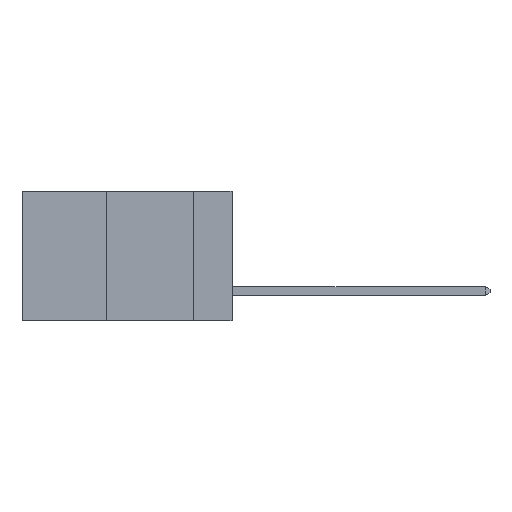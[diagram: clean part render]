
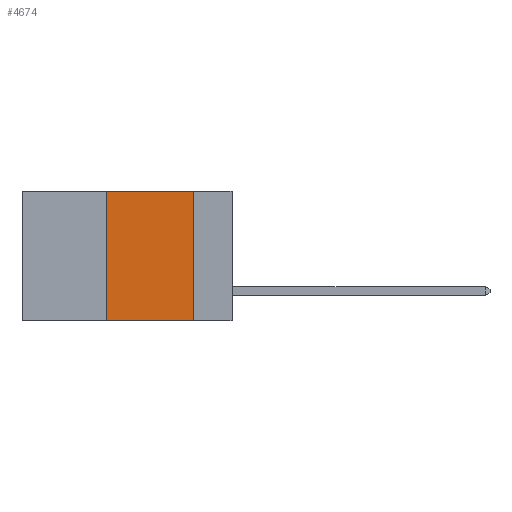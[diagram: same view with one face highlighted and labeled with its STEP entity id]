
A CAD part, left-side view. The second image highlights one B-rep face of the part: STEP entity #4674.
In plain terms, the highlighted planar face has unit normal (-1, 0, 0).
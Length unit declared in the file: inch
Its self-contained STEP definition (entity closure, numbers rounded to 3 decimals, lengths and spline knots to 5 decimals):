
#524 = VECTOR ( 'NONE', #16041, 39.37008 ) ;
#642 = EDGE_CURVE ( 'NONE', #1489, #13528, #15472, .T. ) ;
#1094 = EDGE_LOOP ( 'NONE', ( #17589, #17293, #4717, #20922 ) ) ;
#1489 = VERTEX_POINT ( 'NONE', #21468 ) ;
#2473 = AXIS2_PLACEMENT_3D ( 'NONE', #7374, #22878, #11309 ) ;
#3033 = CARTESIAN_POINT ( 'NONE',  ( 0., 0.36, 0. ) ) ;
#4674 = ADVANCED_FACE ( 'NONE', ( #10718 ), #20958, .F. ) ;
#4717 = ORIENTED_EDGE ( 'NONE', *, *, #10222, .F. ) ;
#4880 = CARTESIAN_POINT ( 'NONE',  ( 0., 0.36, 0. ) ) ;
#4892 = CARTESIAN_POINT ( 'NONE',  ( 0., 0.11, 0. ) ) ;
#5175 = VERTEX_POINT ( 'NONE', #4880 ) ;
#5497 = LINE ( 'NONE', #3033, #10768 ) ;
#5903 = LINE ( 'NONE', #14131, #524 ) ;
#7374 = CARTESIAN_POINT ( 'NONE',  ( 0., 0.6, 0. ) ) ;
#8728 = EDGE_CURVE ( 'NONE', #5175, #10208, #5903, .T. ) ;
#8800 = LINE ( 'NONE', #15427, #13407 ) ;
#9700 = VECTOR ( 'NONE', #23772, 39.37008 ) ;
#10208 = VERTEX_POINT ( 'NONE', #4892 ) ;
#10222 = EDGE_CURVE ( 'NONE', #1489, #5175, #5497, .T. ) ;
#10718 = FACE_OUTER_BOUND ( 'NONE', #1094, .T. ) ;
#10768 = VECTOR ( 'NONE', #14893, 39.37008 ) ;
#11309 = DIRECTION ( 'NONE',  ( 0., 0., -1. ) ) ;
#11674 = DIRECTION ( 'NONE',  ( 0., 0., -1. ) ) ;
#13407 = VECTOR ( 'NONE', #11674, 39.37008 ) ;
#13528 = VERTEX_POINT ( 'NONE', #15564 ) ;
#14131 = CARTESIAN_POINT ( 'NONE',  ( 0., 0.6, 0. ) ) ;
#14893 = DIRECTION ( 'NONE',  ( 0., 0., 1. ) ) ;
#15427 = CARTESIAN_POINT ( 'NONE',  ( 0., 0.11, 0. ) ) ;
#15445 = EDGE_CURVE ( 'NONE', #10208, #13528, #8800, .T. ) ;
#15472 = LINE ( 'NONE', #23644, #9700 ) ;
#15564 = CARTESIAN_POINT ( 'NONE',  ( 0., 0.11, -0.37 ) ) ;
#16041 = DIRECTION ( 'NONE',  ( 0., -1., 0. ) ) ;
#17293 = ORIENTED_EDGE ( 'NONE', *, *, #8728, .F. ) ;
#17589 = ORIENTED_EDGE ( 'NONE', *, *, #15445, .F. ) ;
#20922 = ORIENTED_EDGE ( 'NONE', *, *, #642, .T. ) ;
#20958 = PLANE ( 'NONE',  #2473 ) ;
#21468 = CARTESIAN_POINT ( 'NONE',  ( 0., 0.36, -0.37 ) ) ;
#22878 = DIRECTION ( 'NONE',  ( 1., 0., 0. ) ) ;
#23644 = CARTESIAN_POINT ( 'NONE',  ( 0., 0.6, -0.37 ) ) ;
#23772 = DIRECTION ( 'NONE',  ( 0., -1., 0. ) ) ;
